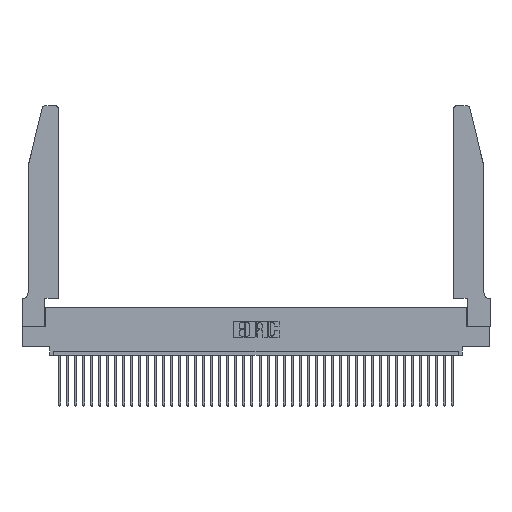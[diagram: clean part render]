
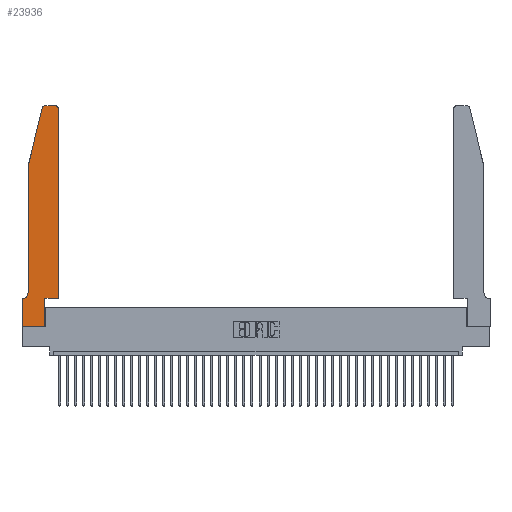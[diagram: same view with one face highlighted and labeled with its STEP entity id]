
A CAD part, top view. The second image highlights one B-rep face of the part: STEP entity #23936.
In plain terms, the highlighted planar face has unit normal (0, 0, 1).
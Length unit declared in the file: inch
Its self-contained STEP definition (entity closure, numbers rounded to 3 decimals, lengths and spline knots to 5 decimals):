
#19 = DIRECTION ( 'NONE',  ( 1., 0., 0. ) ) ;
#528 = CARTESIAN_POINT ( 'NONE',  ( 0., 0.35, 0.37 ) ) ;
#1582 = DIRECTION ( 'NONE',  ( -1., 0., 0. ) ) ;
#2128 = DIRECTION ( 'NONE',  ( 0., 0., 1. ) ) ;
#2439 = VERTEX_POINT ( 'NONE', #21659 ) ;
#2678 = CARTESIAN_POINT ( 'NONE',  ( 0.0755, 2., 0.37 ) ) ;
#2819 = CARTESIAN_POINT ( 'NONE',  ( 0.4505, 0.35, 0.37 ) ) ;
#2863 = VERTEX_POINT ( 'NONE', #4173 ) ;
#3634 = VECTOR ( 'NONE', #10270, 39.37008 ) ;
#4173 = CARTESIAN_POINT ( 'NONE',  ( 0., 0., 0.37 ) ) ;
#4482 = DIRECTION ( 'NONE',  ( -1., 0., 0. ) ) ;
#4933 = CARTESIAN_POINT ( 'NONE',  ( 0.284, 2.72, 0.37 ) ) ;
#5131 = CARTESIAN_POINT ( 'NONE',  ( 0.25487, 2.72718, 0.37 ) ) ;
#6014 = CARTESIAN_POINT ( 'NONE',  ( 0.0055, 0.35, 0.37 ) ) ;
#6094 = CIRCLE ( 'NONE', #19659, 0.07 ) ;
#6846 = DIRECTION ( 'NONE',  ( 0., 1., 0. ) ) ;
#7198 = LINE ( 'NONE', #2678, #25706 ) ;
#7238 = LINE ( 'NONE', #27134, #40259 ) ;
#7284 = AXIS2_PLACEMENT_3D ( 'NONE', #4933, #30809, #21294 ) ;
#7616 = AXIS2_PLACEMENT_3D ( 'NONE', #9033, #2128, #40567 ) ;
#7710 = LINE ( 'NONE', #40127, #33184 ) ;
#7816 = VERTEX_POINT ( 'NONE', #21194 ) ;
#8110 = EDGE_CURVE ( 'NONE', #2863, #2439, #7710, .T. ) ;
#8169 = CARTESIAN_POINT ( 'NONE',  ( 0.0055, 0.42, 0.37 ) ) ;
#9033 = CARTESIAN_POINT ( 'NONE',  ( 0., 0.35, 0.37 ) ) ;
#9545 = EDGE_CURVE ( 'NONE', #41029, #16200, #32369, .T. ) ;
#9608 = VERTEX_POINT ( 'NONE', #5131 ) ;
#10131 = CARTESIAN_POINT ( 'NONE',  ( 0.2865, 0.35, 0.37 ) ) ;
#10270 = DIRECTION ( 'NONE',  ( 0., 1., 0. ) ) ;
#10420 = LINE ( 'NONE', #2819, #40936 ) ;
#10570 = CARTESIAN_POINT ( 'NONE',  ( 0.0755, 0.35, 0.37 ) ) ;
#11710 = EDGE_LOOP ( 'NONE', ( #18828, #30788, #33660, #33255, #36100, #18221, #28572, #38538, #18079, #41047, #32034, #19512 ) ) ;
#12539 = VECTOR ( 'NONE', #34776, 39.37008 ) ;
#12640 = CARTESIAN_POINT ( 'NONE',  ( 0.0755, 0.42, 0.37 ) ) ;
#13808 = VECTOR ( 'NONE', #6846, 39.37008 ) ;
#13842 = EDGE_CURVE ( 'NONE', #16200, #2863, #28514, .T. ) ;
#14384 = EDGE_CURVE ( 'NONE', #20476, #34767, #37467, .T. ) ;
#14578 = DIRECTION ( 'NONE',  ( 0., 0., -1. ) ) ;
#16200 = VERTEX_POINT ( 'NONE', #528 ) ;
#16325 = LINE ( 'NONE', #16608, #13808 ) ;
#16608 = CARTESIAN_POINT ( 'NONE',  ( 0.4505, 0.35, 0.37 ) ) ;
#16691 = CIRCLE ( 'NONE', #23306, 0.03 ) ;
#16843 = VERTEX_POINT ( 'NONE', #23914 ) ;
#17315 = VERTEX_POINT ( 'NONE', #21740 ) ;
#17487 = VERTEX_POINT ( 'NONE', #30365 ) ;
#17968 = DIRECTION ( 'NONE',  ( 0., -1., 0. ) ) ;
#18079 = ORIENTED_EDGE ( 'NONE', *, *, #22712, .T. ) ;
#18103 = FACE_OUTER_BOUND ( 'NONE', #11710, .T. ) ;
#18221 = ORIENTED_EDGE ( 'NONE', *, *, #9545, .T. ) ;
#18828 = ORIENTED_EDGE ( 'NONE', *, *, #38003, .T. ) ;
#19512 = ORIENTED_EDGE ( 'NONE', *, *, #38296, .T. ) ;
#19659 = AXIS2_PLACEMENT_3D ( 'NONE', #8169, #14578, #4482 ) ;
#19839 = VERTEX_POINT ( 'NONE', #19971 ) ;
#19971 = CARTESIAN_POINT ( 'NONE',  ( 0.2865, 0.35, 0.37 ) ) ;
#20464 = DIRECTION ( 'NONE',  ( -1., 0., 0. ) ) ;
#20476 = VERTEX_POINT ( 'NONE', #36377 ) ;
#21194 = CARTESIAN_POINT ( 'NONE',  ( 0.4505, 2.72, 0.37 ) ) ;
#21294 = DIRECTION ( 'NONE',  ( 1., 0., 0. ) ) ;
#21469 = EDGE_CURVE ( 'NONE', #19839, #16843, #10420, .T. ) ;
#21659 = CARTESIAN_POINT ( 'NONE',  ( 0.2865, 0., 0.37 ) ) ;
#21740 = CARTESIAN_POINT ( 'NONE',  ( 0.284, 2.75, 0.37 ) ) ;
#22712 = EDGE_CURVE ( 'NONE', #2439, #19839, #34667, .T. ) ;
#23306 = AXIS2_PLACEMENT_3D ( 'NONE', #38586, #28809, #19 ) ;
#23439 = VECTOR ( 'NONE', #17968, 39.37008 ) ;
#23767 = EDGE_CURVE ( 'NONE', #34767, #41029, #6094, .T. ) ;
#23914 = CARTESIAN_POINT ( 'NONE',  ( 0.4505, 0.35, 0.37 ) ) ;
#23936 = ADVANCED_FACE ( 'NONE', ( #18103 ), #34275, .T. ) ;
#25555 = CIRCLE ( 'NONE', #7284, 0.03 ) ;
#25706 = VECTOR ( 'NONE', #34949, 39.37008 ) ;
#27079 = EDGE_CURVE ( 'NONE', #16843, #7816, #16325, .T. ) ;
#27097 = DIRECTION ( 'NONE',  ( 1., 0., 0. ) ) ;
#27134 = CARTESIAN_POINT ( 'NONE',  ( 0.2605, 2.75, 0.37 ) ) ;
#28514 = LINE ( 'NONE', #29265, #12539 ) ;
#28572 = ORIENTED_EDGE ( 'NONE', *, *, #13842, .T. ) ;
#28809 = DIRECTION ( 'NONE',  ( 0., 0., 1. ) ) ;
#29265 = CARTESIAN_POINT ( 'NONE',  ( 0., 0., 0.37 ) ) ;
#30365 = CARTESIAN_POINT ( 'NONE',  ( 0.4205, 2.75, 0.37 ) ) ;
#30788 = ORIENTED_EDGE ( 'NONE', *, *, #40576, .T. ) ;
#30809 = DIRECTION ( 'NONE',  ( 0., 0., 1. ) ) ;
#31891 = DIRECTION ( 'NONE',  ( 1., 0., 0. ) ) ;
#32034 = ORIENTED_EDGE ( 'NONE', *, *, #27079, .T. ) ;
#32369 = LINE ( 'NONE', #10570, #38365 ) ;
#33184 = VECTOR ( 'NONE', #27097, 39.37008 ) ;
#33255 = ORIENTED_EDGE ( 'NONE', *, *, #14384, .T. ) ;
#33660 = ORIENTED_EDGE ( 'NONE', *, *, #38775, .T. ) ;
#34275 = PLANE ( 'NONE',  #7616 ) ;
#34667 = LINE ( 'NONE', #10131, #3634 ) ;
#34767 = VERTEX_POINT ( 'NONE', #12640 ) ;
#34776 = DIRECTION ( 'NONE',  ( 0., -1., 0. ) ) ;
#34949 = DIRECTION ( 'NONE',  ( -0.239, -0.971, 0. ) ) ;
#36100 = ORIENTED_EDGE ( 'NONE', *, *, #23767, .T. ) ;
#36377 = CARTESIAN_POINT ( 'NONE',  ( 0.0755, 2., 0.37 ) ) ;
#37467 = LINE ( 'NONE', #38217, #23439 ) ;
#38003 = EDGE_CURVE ( 'NONE', #17487, #17315, #7238, .T. ) ;
#38217 = CARTESIAN_POINT ( 'NONE',  ( 0.0755, 2., 0.37 ) ) ;
#38296 = EDGE_CURVE ( 'NONE', #7816, #17487, #16691, .T. ) ;
#38365 = VECTOR ( 'NONE', #20464, 39.37008 ) ;
#38538 = ORIENTED_EDGE ( 'NONE', *, *, #8110, .T. ) ;
#38586 = CARTESIAN_POINT ( 'NONE',  ( 0.4205, 2.72, 0.37 ) ) ;
#38775 = EDGE_CURVE ( 'NONE', #9608, #20476, #7198, .T. ) ;
#40127 = CARTESIAN_POINT ( 'NONE',  ( 0., 0., 0.37 ) ) ;
#40259 = VECTOR ( 'NONE', #1582, 39.37008 ) ;
#40567 = DIRECTION ( 'NONE',  ( 1., 0., 0. ) ) ;
#40576 = EDGE_CURVE ( 'NONE', #17315, #9608, #25555, .T. ) ;
#40936 = VECTOR ( 'NONE', #31891, 39.37008 ) ;
#41029 = VERTEX_POINT ( 'NONE', #6014 ) ;
#41047 = ORIENTED_EDGE ( 'NONE', *, *, #21469, .T. ) ;
